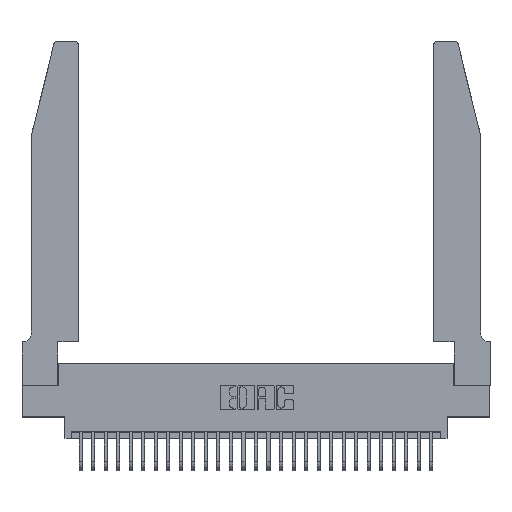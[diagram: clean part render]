
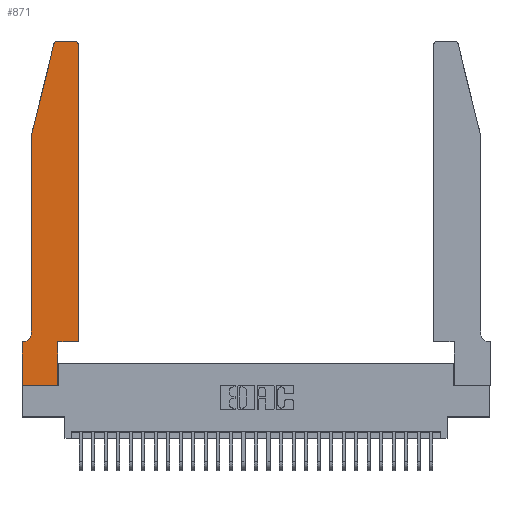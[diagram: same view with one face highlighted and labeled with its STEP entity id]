
A CAD part, top view. The second image highlights one B-rep face of the part: STEP entity #871.
In plain terms, the highlighted planar face has unit normal (0, 0, 1).
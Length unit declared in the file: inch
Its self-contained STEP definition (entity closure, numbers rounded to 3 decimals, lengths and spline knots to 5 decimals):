
#230 = CARTESIAN_POINT ( 'NONE',  ( 0., 0.35, 0.37 ) ) ;
#307 = EDGE_CURVE ( 'NONE', #27576, #19155, #15272, .T. ) ;
#486 = EDGE_CURVE ( 'NONE', #26423, #30143, #17126, .T. ) ;
#842 = VECTOR ( 'NONE', #24288, 39.37008 ) ;
#871 = ADVANCED_FACE ( 'NONE', ( #13769 ), #2001, .T. ) ;
#951 = EDGE_CURVE ( 'NONE', #11430, #7331, #24096, .T. ) ;
#978 = ORIENTED_EDGE ( 'NONE', *, *, #31043, .T. ) ;
#1648 = CARTESIAN_POINT ( 'NONE',  ( 0.2865, 0., 0.37 ) ) ;
#1842 = DIRECTION ( 'NONE',  ( 1., 0., 0. ) ) ;
#1882 = DIRECTION ( 'NONE',  ( 0., 0., 1. ) ) ;
#2001 = PLANE ( 'NONE',  #18818 ) ;
#2190 = DIRECTION ( 'NONE',  ( 0., 1., 0. ) ) ;
#2294 = LINE ( 'NONE', #10773, #20722 ) ;
#2613 = CARTESIAN_POINT ( 'NONE',  ( 0.284, 2.72, 0.37 ) ) ;
#2783 = DIRECTION ( 'NONE',  ( 0., -1., 0. ) ) ;
#2832 = CARTESIAN_POINT ( 'NONE',  ( 0.0055, 0.35, 0.37 ) ) ;
#3039 = ORIENTED_EDGE ( 'NONE', *, *, #4564, .T. ) ;
#3440 = ORIENTED_EDGE ( 'NONE', *, *, #21557, .T. ) ;
#3649 = ORIENTED_EDGE ( 'NONE', *, *, #486, .T. ) ;
#4187 = CARTESIAN_POINT ( 'NONE',  ( 0.284, 2.75, 0.37 ) ) ;
#4276 = CARTESIAN_POINT ( 'NONE',  ( 0., 0., 0.37 ) ) ;
#4326 = CARTESIAN_POINT ( 'NONE',  ( 0.0755, 2., 0.37 ) ) ;
#4422 = CARTESIAN_POINT ( 'NONE',  ( 0., 0., 0.37 ) ) ;
#4501 = ORIENTED_EDGE ( 'NONE', *, *, #15985, .T. ) ;
#4564 = EDGE_CURVE ( 'NONE', #9045, #11430, #10367, .T. ) ;
#5130 = CARTESIAN_POINT ( 'NONE',  ( 0.0055, 0.42, 0.37 ) ) ;
#5152 = DIRECTION ( 'NONE',  ( 1., 0., 0. ) ) ;
#5396 = CARTESIAN_POINT ( 'NONE',  ( 0.4205, 2.75, 0.37 ) ) ;
#5701 = CIRCLE ( 'NONE', #6367, 0.03 ) ;
#6259 = DIRECTION ( 'NONE',  ( 0., -1., 0. ) ) ;
#6367 = AXIS2_PLACEMENT_3D ( 'NONE', #2613, #19452, #5152 ) ;
#7331 = VERTEX_POINT ( 'NONE', #4187 ) ;
#7428 = EDGE_CURVE ( 'NONE', #9846, #9045, #15807, .T. ) ;
#7546 = EDGE_CURVE ( 'NONE', #7331, #11952, #5701, .T. ) ;
#7567 = DIRECTION ( 'NONE',  ( -1., 0., 0. ) ) ;
#8675 = VECTOR ( 'NONE', #2190, 39.37008 ) ;
#9045 = VERTEX_POINT ( 'NONE', #26173 ) ;
#9259 = ORIENTED_EDGE ( 'NONE', *, *, #12004, .T. ) ;
#9483 = CARTESIAN_POINT ( 'NONE',  ( 0.4505, 0.35, 0.37 ) ) ;
#9576 = VERTEX_POINT ( 'NONE', #1648 ) ;
#9846 = VERTEX_POINT ( 'NONE', #25068 ) ;
#10367 = CIRCLE ( 'NONE', #25619, 0.03 ) ;
#10518 = VECTOR ( 'NONE', #20504, 39.37008 ) ;
#10643 = DIRECTION ( 'NONE',  ( 0., 1., 0. ) ) ;
#10765 = VECTOR ( 'NONE', #2783, 39.37008 ) ;
#10773 = CARTESIAN_POINT ( 'NONE',  ( 0.0755, 2., 0.37 ) ) ;
#10807 = CARTESIAN_POINT ( 'NONE',  ( 0.4505, 0.35, 0.37 ) ) ;
#11430 = VERTEX_POINT ( 'NONE', #5396 ) ;
#11498 = VECTOR ( 'NONE', #16117, 39.37008 ) ;
#11872 = DIRECTION ( 'NONE',  ( 0., 0., 1. ) ) ;
#11952 = VERTEX_POINT ( 'NONE', #21488 ) ;
#12004 = EDGE_CURVE ( 'NONE', #19155, #26205, #29736, .T. ) ;
#13186 = DIRECTION ( 'NONE',  ( -0.239, -0.971, 0. ) ) ;
#13562 = CARTESIAN_POINT ( 'NONE',  ( 0., 0.35, 0.37 ) ) ;
#13769 = FACE_OUTER_BOUND ( 'NONE', #26573, .T. ) ;
#15272 = LINE ( 'NONE', #4326, #27864 ) ;
#15807 = LINE ( 'NONE', #9483, #8675 ) ;
#15985 = EDGE_CURVE ( 'NONE', #9576, #27685, #22824, .T. ) ;
#16117 = DIRECTION ( 'NONE',  ( -1., 0., 0. ) ) ;
#16572 = VECTOR ( 'NONE', #10643, 39.37008 ) ;
#16594 = ORIENTED_EDGE ( 'NONE', *, *, #7546, .T. ) ;
#17126 = LINE ( 'NONE', #4276, #10765 ) ;
#17625 = ORIENTED_EDGE ( 'NONE', *, *, #27486, .T. ) ;
#17835 = AXIS2_PLACEMENT_3D ( 'NONE', #5130, #21798, #7567 ) ;
#18818 = AXIS2_PLACEMENT_3D ( 'NONE', #230, #1882, #1842 ) ;
#18872 = LINE ( 'NONE', #10807, #25928 ) ;
#19155 = VERTEX_POINT ( 'NONE', #22949 ) ;
#19452 = DIRECTION ( 'NONE',  ( 0., 0., 1. ) ) ;
#20504 = DIRECTION ( 'NONE',  ( -1., 0., 0. ) ) ;
#20722 = VECTOR ( 'NONE', #13186, 39.37008 ) ;
#21315 = CARTESIAN_POINT ( 'NONE',  ( 0.2605, 2.75, 0.37 ) ) ;
#21488 = CARTESIAN_POINT ( 'NONE',  ( 0.25487, 2.72718, 0.37 ) ) ;
#21491 = ORIENTED_EDGE ( 'NONE', *, *, #307, .T. ) ;
#21557 = EDGE_CURVE ( 'NONE', #27685, #9846, #18872, .T. ) ;
#21798 = DIRECTION ( 'NONE',  ( 0., 0., -1. ) ) ;
#21885 = CARTESIAN_POINT ( 'NONE',  ( 0., 0., 0.37 ) ) ;
#22603 = ORIENTED_EDGE ( 'NONE', *, *, #30032, .T. ) ;
#22824 = LINE ( 'NONE', #29513, #16572 ) ;
#22949 = CARTESIAN_POINT ( 'NONE',  ( 0.0755, 0.42, 0.37 ) ) ;
#24096 = LINE ( 'NONE', #21315, #11498 ) ;
#24288 = DIRECTION ( 'NONE',  ( 1., 0., 0. ) ) ;
#25028 = DIRECTION ( 'NONE',  ( 1., 0., 0. ) ) ;
#25068 = CARTESIAN_POINT ( 'NONE',  ( 0.4505, 0.35, 0.37 ) ) ;
#25619 = AXIS2_PLACEMENT_3D ( 'NONE', #26095, #11872, #28432 ) ;
#25902 = ORIENTED_EDGE ( 'NONE', *, *, #951, .T. ) ;
#25928 = VECTOR ( 'NONE', #25028, 39.37008 ) ;
#26095 = CARTESIAN_POINT ( 'NONE',  ( 0.4205, 2.72, 0.37 ) ) ;
#26173 = CARTESIAN_POINT ( 'NONE',  ( 0.4505, 2.72, 0.37 ) ) ;
#26205 = VERTEX_POINT ( 'NONE', #2832 ) ;
#26423 = VERTEX_POINT ( 'NONE', #13562 ) ;
#26448 = LINE ( 'NONE', #21885, #842 ) ;
#26573 = EDGE_LOOP ( 'NONE', ( #25902, #16594, #17625, #21491, #9259, #22603, #3649, #978, #4501, #3440, #30782, #3039 ) ) ;
#27486 = EDGE_CURVE ( 'NONE', #11952, #27576, #2294, .T. ) ;
#27576 = VERTEX_POINT ( 'NONE', #30040 ) ;
#27685 = VERTEX_POINT ( 'NONE', #28084 ) ;
#27864 = VECTOR ( 'NONE', #6259, 39.37008 ) ;
#28084 = CARTESIAN_POINT ( 'NONE',  ( 0.2865, 0.35, 0.37 ) ) ;
#28432 = DIRECTION ( 'NONE',  ( 1., 0., 0. ) ) ;
#29513 = CARTESIAN_POINT ( 'NONE',  ( 0.2865, 0.35, 0.37 ) ) ;
#29736 = CIRCLE ( 'NONE', #17835, 0.07 ) ;
#29932 = CARTESIAN_POINT ( 'NONE',  ( 0.0755, 0.35, 0.37 ) ) ;
#30032 = EDGE_CURVE ( 'NONE', #26205, #26423, #30177, .T. ) ;
#30040 = CARTESIAN_POINT ( 'NONE',  ( 0.0755, 2., 0.37 ) ) ;
#30143 = VERTEX_POINT ( 'NONE', #4422 ) ;
#30177 = LINE ( 'NONE', #29932, #10518 ) ;
#30782 = ORIENTED_EDGE ( 'NONE', *, *, #7428, .T. ) ;
#31043 = EDGE_CURVE ( 'NONE', #30143, #9576, #26448, .T. ) ;
